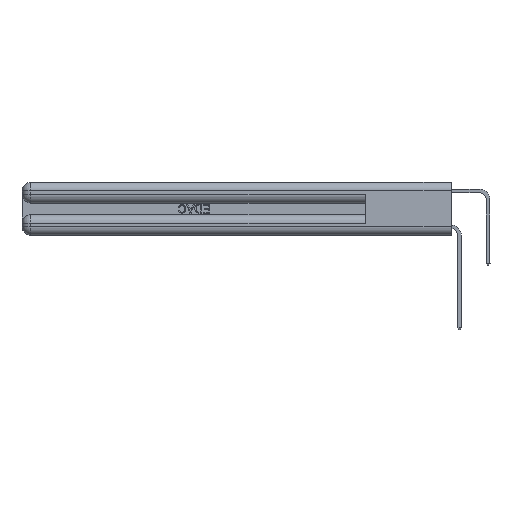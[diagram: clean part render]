
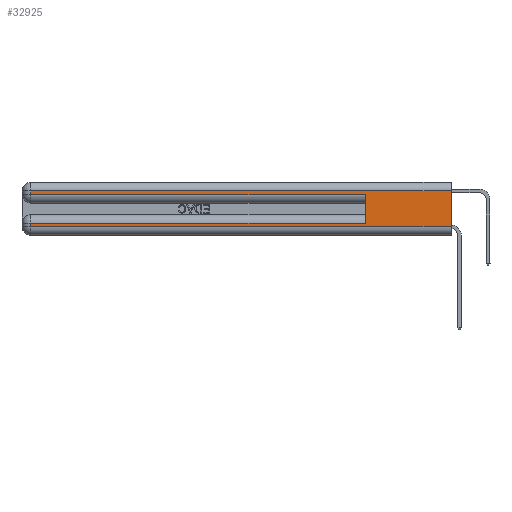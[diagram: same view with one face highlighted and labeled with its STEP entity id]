
A CAD part, left-side view. The second image highlights one B-rep face of the part: STEP entity #32925.
In plain terms, the highlighted planar face has unit normal (-1, 0, 0).
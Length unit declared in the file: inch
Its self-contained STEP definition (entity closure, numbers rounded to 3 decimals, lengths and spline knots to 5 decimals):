
#1254 = CARTESIAN_POINT ( 'NONE',  ( 0., 2.94, 0.285 ) ) ;
#1797 = EDGE_CURVE ( 'NONE', #2925, #12972, #15643, .T. ) ;
#2085 = CARTESIAN_POINT ( 'NONE',  ( 0., 0.6, 0.285 ) ) ;
#2347 = ORIENTED_EDGE ( 'NONE', *, *, #1797, .F. ) ;
#2763 = LINE ( 'NONE', #5487, #18933 ) ;
#2925 = VERTEX_POINT ( 'NONE', #7157 ) ;
#3021 = LINE ( 'NONE', #23802, #31270 ) ;
#3788 = VERTEX_POINT ( 'NONE', #30088 ) ;
#4525 = LINE ( 'NONE', #22733, #25078 ) ;
#4577 = DIRECTION ( 'NONE',  ( 0., -1., 0. ) ) ;
#4807 = CARTESIAN_POINT ( 'NONE',  ( 0., 0., 0.06 ) ) ;
#5327 = DIRECTION ( 'NONE',  ( 0., 0., -1. ) ) ;
#5487 = CARTESIAN_POINT ( 'NONE',  ( 0., 0., 0.31 ) ) ;
#5774 = VERTEX_POINT ( 'NONE', #16833 ) ;
#6837 = AXIS2_PLACEMENT_3D ( 'NONE', #7944, #23147, #25989 ) ;
#7157 = CARTESIAN_POINT ( 'NONE',  ( 0., 0.6, 0.085 ) ) ;
#7281 = VERTEX_POINT ( 'NONE', #20970 ) ;
#7942 = EDGE_CURVE ( 'NONE', #30933, #28652, #3021, .T. ) ;
#7944 = CARTESIAN_POINT ( 'NONE',  ( 0., 0., 0.37 ) ) ;
#8035 = ORIENTED_EDGE ( 'NONE', *, *, #19887, .T. ) ;
#8844 = DIRECTION ( 'NONE',  ( 0., 0., -1. ) ) ;
#9539 = DIRECTION ( 'NONE',  ( 0., -1., 0. ) ) ;
#10089 = VERTEX_POINT ( 'NONE', #32375 ) ;
#11946 = CARTESIAN_POINT ( 'NONE',  ( 0., 2.94, 0.31 ) ) ;
#12791 = PLANE ( 'NONE',  #6837 ) ;
#12972 = VERTEX_POINT ( 'NONE', #2085 ) ;
#13938 = VECTOR ( 'NONE', #9539, 39.37008 ) ;
#14439 = VECTOR ( 'NONE', #23771, 39.37008 ) ;
#15096 = ORIENTED_EDGE ( 'NONE', *, *, #31745, .T. ) ;
#15240 = CARTESIAN_POINT ( 'NONE',  ( 0., 2.94, 0.37 ) ) ;
#15310 = EDGE_CURVE ( 'NONE', #28652, #12972, #20048, .T. ) ;
#15643 = LINE ( 'NONE', #22658, #14439 ) ;
#15854 = DIRECTION ( 'NONE',  ( 0., 1., 0. ) ) ;
#15950 = ORIENTED_EDGE ( 'NONE', *, *, #30650, .T. ) ;
#16529 = FACE_OUTER_BOUND ( 'NONE', #32826, .T. ) ;
#16833 = CARTESIAN_POINT ( 'NONE',  ( 0., 0., 0.31 ) ) ;
#17449 = VECTOR ( 'NONE', #15854, 39.37008 ) ;
#17908 = LINE ( 'NONE', #15240, #30814 ) ;
#18661 = EDGE_CURVE ( 'NONE', #3788, #10089, #32309, .T. ) ;
#18680 = ORIENTED_EDGE ( 'NONE', *, *, #7942, .T. ) ;
#18933 = VECTOR ( 'NONE', #20942, 39.37008 ) ;
#19887 = EDGE_CURVE ( 'NONE', #5774, #30933, #2763, .T. ) ;
#20048 = LINE ( 'NONE', #32937, #13938 ) ;
#20942 = DIRECTION ( 'NONE',  ( 0., 1., 0. ) ) ;
#20970 = CARTESIAN_POINT ( 'NONE',  ( 0., 2.94, 0.085 ) ) ;
#21373 = ORIENTED_EDGE ( 'NONE', *, *, #22002, .F. ) ;
#22002 = EDGE_CURVE ( 'NONE', #5774, #10089, #4525, .T. ) ;
#22658 = CARTESIAN_POINT ( 'NONE',  ( 0., 0.6, 0.145 ) ) ;
#22733 = CARTESIAN_POINT ( 'NONE',  ( 0., 0., 0.37 ) ) ;
#23147 = DIRECTION ( 'NONE',  ( 1., 0., 0. ) ) ;
#23771 = DIRECTION ( 'NONE',  ( 0., 0., 1. ) ) ;
#23802 = CARTESIAN_POINT ( 'NONE',  ( 0., 2.94, 0.37 ) ) ;
#25078 = VECTOR ( 'NONE', #26017, 39.37008 ) ;
#25455 = VECTOR ( 'NONE', #4577, 39.37008 ) ;
#25727 = ORIENTED_EDGE ( 'NONE', *, *, #15310, .T. ) ;
#25989 = DIRECTION ( 'NONE',  ( 0., 0., -1. ) ) ;
#26017 = DIRECTION ( 'NONE',  ( 0., 0., -1. ) ) ;
#26097 = CARTESIAN_POINT ( 'NONE',  ( 0., 0., 0.085 ) ) ;
#28060 = ORIENTED_EDGE ( 'NONE', *, *, #18661, .T. ) ;
#28652 = VERTEX_POINT ( 'NONE', #1254 ) ;
#30088 = CARTESIAN_POINT ( 'NONE',  ( 0., 2.94, 0.06 ) ) ;
#30650 = EDGE_CURVE ( 'NONE', #7281, #3788, #17908, .T. ) ;
#30814 = VECTOR ( 'NONE', #5327, 39.37008 ) ;
#30933 = VERTEX_POINT ( 'NONE', #11946 ) ;
#31145 = LINE ( 'NONE', #26097, #17449 ) ;
#31270 = VECTOR ( 'NONE', #8844, 39.37008 ) ;
#31745 = EDGE_CURVE ( 'NONE', #2925, #7281, #31145, .T. ) ;
#32309 = LINE ( 'NONE', #4807, #25455 ) ;
#32375 = CARTESIAN_POINT ( 'NONE',  ( 0., 0., 0.06 ) ) ;
#32826 = EDGE_LOOP ( 'NONE', ( #21373, #8035, #18680, #25727, #2347, #15096, #15950, #28060 ) ) ;
#32925 = ADVANCED_FACE ( 'NONE', ( #16529 ), #12791, .F. ) ;
#32937 = CARTESIAN_POINT ( 'NONE',  ( 0., 0., 0.285 ) ) ;
